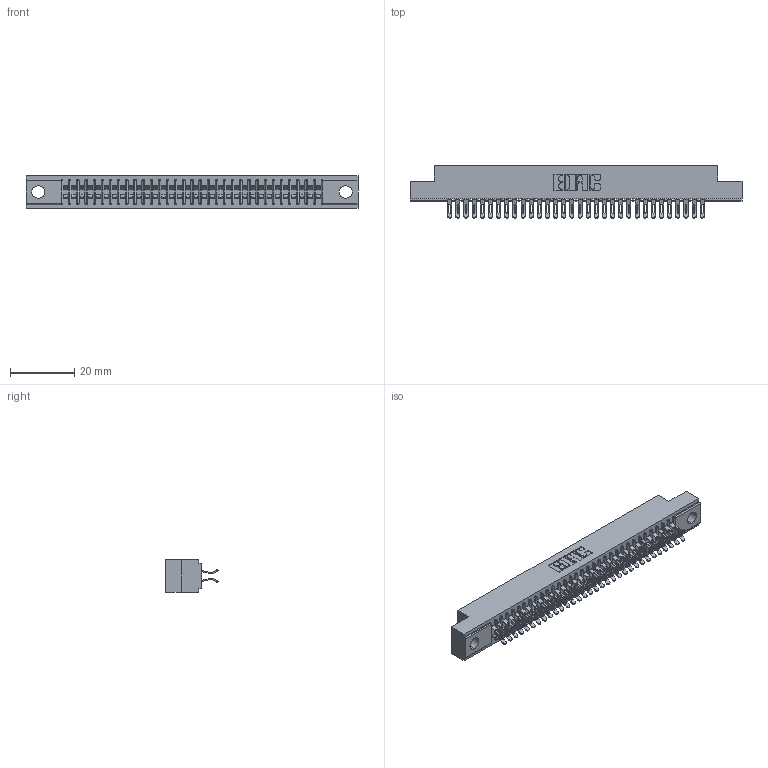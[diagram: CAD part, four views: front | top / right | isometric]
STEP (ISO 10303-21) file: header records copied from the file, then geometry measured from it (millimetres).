
FILE_DESCRIPTION (( 'STEP AP203' ), '1' );
FILE_NAME ('341-064-555-204.STEP', '2018-08-07T18:22:38', ( '' ), ( '' ), 'SwSTEP 2.0', 'SolidWorks 2016', '' );
FILE_SCHEMA (( 'CONFIG_CONTROL_DESIGN' ));
Length unit declared in the file: inch
Products named in the file (3): 341 Part_.156 (3.96) Dia Mounting Holes; 341-292-001_341-292-155; 341-064-555-204
Assembly tree (65 placements, depth 2):
  341-064-555-204
    341 Part_.156 (3.96) Dia Mounting Holes
    341-292-001_341-292-155  x64
Bounding box: 103.5 x 16.31 x 10.16 mm (x, y, z)
Volume: 7609.9 mm3; surface area: 13601.5 mm2
Topology: 65 solids, 65 shells, 5122 faces, 15296 edges, 9958 vertices
Faces by surface type: plane 2770, cylinder 2224, sphere 66, torus 62
Entity records: 40947 total; most frequent: CARTESIAN_POINT 6828, ORIENTED_EDGE 6772, DIRECTION 6616, EDGE_CURVE 3386, VECTOR 2716, LINE 2716, VERTEX_POINT 2146, AXIS2_PLACEMENT_3D 1950
